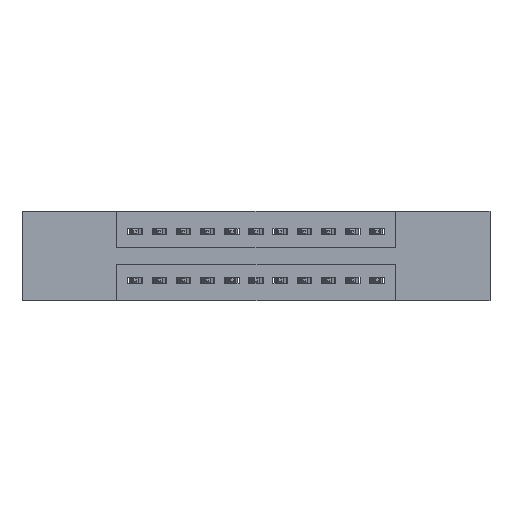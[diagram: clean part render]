
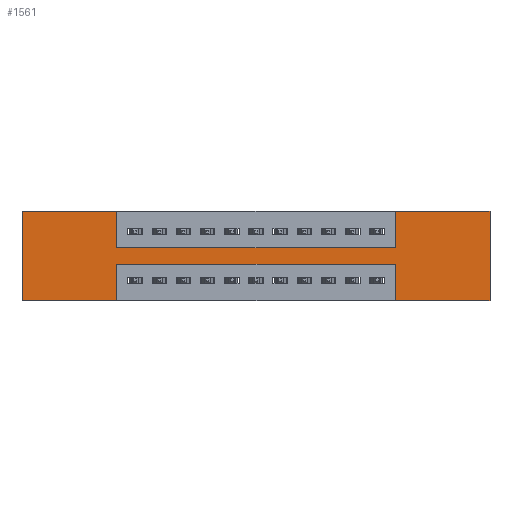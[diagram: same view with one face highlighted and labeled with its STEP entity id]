
A CAD part, front view. The second image highlights one B-rep face of the part: STEP entity #1561.
In plain terms, the highlighted planar face has unit normal (0, -1, 0).
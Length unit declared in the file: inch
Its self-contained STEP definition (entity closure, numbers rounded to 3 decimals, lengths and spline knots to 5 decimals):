
#7 = VECTOR ( 'NONE', #11554, 39.37008 ) ;
#179 = VERTEX_POINT ( 'NONE', #7633 ) ;
#511 = EDGE_CURVE ( 'NONE', #4056, #7003, #1704, .T. ) ;
#553 = ORIENTED_EDGE ( 'NONE', *, *, #4431, .F. ) ;
#593 = CARTESIAN_POINT ( 'NONE',  ( 0.3925, 0., -0.22 ) ) ;
#606 = DIRECTION ( 'NONE',  ( -1., 0., 0. ) ) ;
#780 = ORIENTED_EDGE ( 'NONE', *, *, #12172, .F. ) ;
#956 = CARTESIAN_POINT ( 'NONE',  ( 0.3925, 0., -0.15 ) ) ;
#1561 = ADVANCED_FACE ( 'NONE', ( #12378 ), #12364, .T. ) ;
#1682 = CARTESIAN_POINT ( 'NONE',  ( 0., 0., -0.37 ) ) ;
#1704 = LINE ( 'NONE', #2734, #11685 ) ;
#1779 = CARTESIAN_POINT ( 'NONE',  ( 1.5425, 0., -0.37 ) ) ;
#1847 = ORIENTED_EDGE ( 'NONE', *, *, #8755, .F. ) ;
#1900 = VERTEX_POINT ( 'NONE', #8510 ) ;
#1908 = EDGE_LOOP ( 'NONE', ( #553, #780, #9632, #12786, #6740, #9079, #8675, #1847, #7963, #3435, #7189, #1911 ) ) ;
#1911 = ORIENTED_EDGE ( 'NONE', *, *, #2540, .F. ) ;
#1969 = DIRECTION ( 'NONE',  ( -1., 0., 0. ) ) ;
#2091 = CARTESIAN_POINT ( 'NONE',  ( 0., 0., 0. ) ) ;
#2323 = EDGE_CURVE ( 'NONE', #179, #4056, #6180, .T. ) ;
#2452 = LINE ( 'NONE', #956, #12347 ) ;
#2473 = VERTEX_POINT ( 'NONE', #593 ) ;
#2540 = EDGE_CURVE ( 'NONE', #4148, #3386, #6337, .T. ) ;
#2588 = VERTEX_POINT ( 'NONE', #7900 ) ;
#2734 = CARTESIAN_POINT ( 'NONE',  ( 0.3925, 0., 0. ) ) ;
#3368 = VECTOR ( 'NONE', #8095, 39.37008 ) ;
#3386 = VERTEX_POINT ( 'NONE', #11928 ) ;
#3404 = EDGE_CURVE ( 'NONE', #6036, #9484, #6170, .T. ) ;
#3435 = ORIENTED_EDGE ( 'NONE', *, *, #2323, .F. ) ;
#3531 = VECTOR ( 'NONE', #606, 39.37008 ) ;
#3723 = CARTESIAN_POINT ( 'NONE',  ( 1.5425, 0., 0. ) ) ;
#3752 = DIRECTION ( 'NONE',  ( 0., 0., 1. ) ) ;
#3759 = DIRECTION ( 'NONE',  ( -1., 0., 0. ) ) ;
#3763 = DIRECTION ( 'NONE',  ( 0., 0., 1. ) ) ;
#4056 = VERTEX_POINT ( 'NONE', #6057 ) ;
#4084 = CARTESIAN_POINT ( 'NONE',  ( 0.3925, 0., -0.15 ) ) ;
#4148 = VERTEX_POINT ( 'NONE', #8614 ) ;
#4316 = LINE ( 'NONE', #7426, #9154 ) ;
#4431 = EDGE_CURVE ( 'NONE', #2473, #4148, #5501, .T. ) ;
#4514 = EDGE_CURVE ( 'NONE', #11190, #1900, #9906, .T. ) ;
#4604 = DIRECTION ( 'NONE',  ( 0., 0., -1. ) ) ;
#4833 = EDGE_CURVE ( 'NONE', #5006, #6036, #4316, .T. ) ;
#5006 = VERTEX_POINT ( 'NONE', #6588 ) ;
#5441 = EDGE_CURVE ( 'NONE', #2588, #5006, #11290, .T. ) ;
#5501 = LINE ( 'NONE', #11503, #7 ) ;
#5519 = DIRECTION ( 'NONE',  ( 1., 0., 0. ) ) ;
#5631 = EDGE_CURVE ( 'NONE', #3386, #179, #6920, .T. ) ;
#5776 = CARTESIAN_POINT ( 'NONE',  ( 0., 0., 0. ) ) ;
#5808 = LINE ( 'NONE', #6914, #10753 ) ;
#6036 = VERTEX_POINT ( 'NONE', #6390 ) ;
#6057 = CARTESIAN_POINT ( 'NONE',  ( 0.3925, 0., 0. ) ) ;
#6099 = VECTOR ( 'NONE', #7266, 39.37008 ) ;
#6170 = LINE ( 'NONE', #12039, #3368 ) ;
#6180 = LINE ( 'NONE', #2091, #11639 ) ;
#6283 = LINE ( 'NONE', #12777, #11181 ) ;
#6337 = LINE ( 'NONE', #1682, #3531 ) ;
#6390 = CARTESIAN_POINT ( 'NONE',  ( 1.935, 0., 0. ) ) ;
#6588 = CARTESIAN_POINT ( 'NONE',  ( 1.5425, 0., 0. ) ) ;
#6740 = ORIENTED_EDGE ( 'NONE', *, *, #3404, .F. ) ;
#6914 = CARTESIAN_POINT ( 'NONE',  ( 0.3925, 0., -0.22 ) ) ;
#6920 = LINE ( 'NONE', #5776, #9271 ) ;
#7003 = VERTEX_POINT ( 'NONE', #4084 ) ;
#7137 = DIRECTION ( 'NONE',  ( 1., 0., 0. ) ) ;
#7189 = ORIENTED_EDGE ( 'NONE', *, *, #5631, .F. ) ;
#7266 = DIRECTION ( 'NONE',  ( 0., 0., 1. ) ) ;
#7375 = CARTESIAN_POINT ( 'NONE',  ( 1.5425, 0., -0.37 ) ) ;
#7426 = CARTESIAN_POINT ( 'NONE',  ( 0., 0., 0. ) ) ;
#7633 = CARTESIAN_POINT ( 'NONE',  ( 0., 0., 0. ) ) ;
#7900 = CARTESIAN_POINT ( 'NONE',  ( 1.5425, 0., -0.15 ) ) ;
#7963 = ORIENTED_EDGE ( 'NONE', *, *, #511, .F. ) ;
#8095 = DIRECTION ( 'NONE',  ( 0., 0., -1. ) ) ;
#8510 = CARTESIAN_POINT ( 'NONE',  ( 1.5425, 0., -0.22 ) ) ;
#8606 = DIRECTION ( 'NONE',  ( 1., 0., 0. ) ) ;
#8614 = CARTESIAN_POINT ( 'NONE',  ( 0.3925, 0., -0.37 ) ) ;
#8675 = ORIENTED_EDGE ( 'NONE', *, *, #5441, .F. ) ;
#8755 = EDGE_CURVE ( 'NONE', #7003, #2588, #2452, .T. ) ;
#8913 = AXIS2_PLACEMENT_3D ( 'NONE', #9661, #9701, #4604 ) ;
#9079 = ORIENTED_EDGE ( 'NONE', *, *, #4833, .F. ) ;
#9154 = VECTOR ( 'NONE', #8606, 39.37008 ) ;
#9271 = VECTOR ( 'NONE', #3752, 39.37008 ) ;
#9484 = VERTEX_POINT ( 'NONE', #10529 ) ;
#9620 = VECTOR ( 'NONE', #3763, 39.37008 ) ;
#9632 = ORIENTED_EDGE ( 'NONE', *, *, #4514, .F. ) ;
#9661 = CARTESIAN_POINT ( 'NONE',  ( 0., 0., -0.37 ) ) ;
#9701 = DIRECTION ( 'NONE',  ( 0., -1., 0. ) ) ;
#9906 = LINE ( 'NONE', #1779, #9620 ) ;
#10529 = CARTESIAN_POINT ( 'NONE',  ( 1.935, 0., -0.37 ) ) ;
#10753 = VECTOR ( 'NONE', #3759, 39.37008 ) ;
#11181 = VECTOR ( 'NONE', #1969, 39.37008 ) ;
#11190 = VERTEX_POINT ( 'NONE', #7375 ) ;
#11290 = LINE ( 'NONE', #3723, #6099 ) ;
#11503 = CARTESIAN_POINT ( 'NONE',  ( 0.3925, 0., -0.37 ) ) ;
#11554 = DIRECTION ( 'NONE',  ( 0., 0., -1. ) ) ;
#11639 = VECTOR ( 'NONE', #5519, 39.37008 ) ;
#11685 = VECTOR ( 'NONE', #12495, 39.37008 ) ;
#11928 = CARTESIAN_POINT ( 'NONE',  ( 0., 0., -0.37 ) ) ;
#12039 = CARTESIAN_POINT ( 'NONE',  ( 1.935, 0., 0. ) ) ;
#12172 = EDGE_CURVE ( 'NONE', #1900, #2473, #5808, .T. ) ;
#12310 = EDGE_CURVE ( 'NONE', #9484, #11190, #6283, .T. ) ;
#12347 = VECTOR ( 'NONE', #7137, 39.37008 ) ;
#12364 = PLANE ( 'NONE',  #8913 ) ;
#12378 = FACE_OUTER_BOUND ( 'NONE', #1908, .T. ) ;
#12495 = DIRECTION ( 'NONE',  ( 0., 0., -1. ) ) ;
#12777 = CARTESIAN_POINT ( 'NONE',  ( 0., 0., -0.37 ) ) ;
#12786 = ORIENTED_EDGE ( 'NONE', *, *, #12310, .F. ) ;
